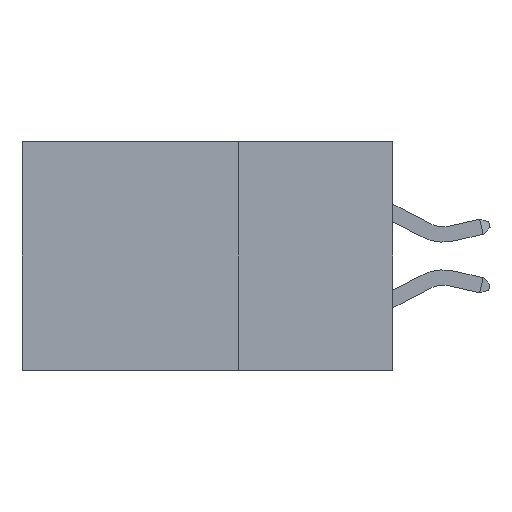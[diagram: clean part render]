
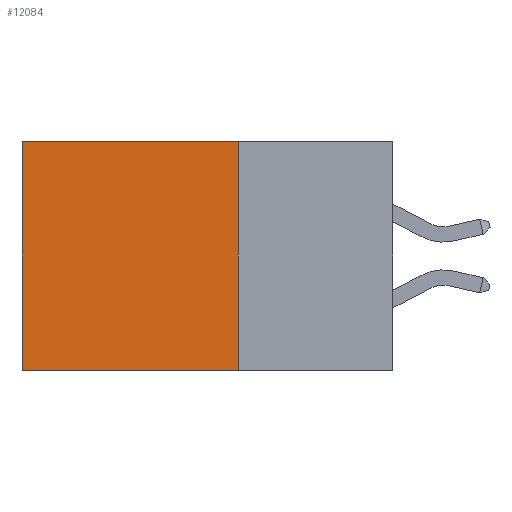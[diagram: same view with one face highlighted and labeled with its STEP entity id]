
A CAD part, left-side view. The second image highlights one B-rep face of the part: STEP entity #12084.
In plain terms, the highlighted planar face has unit normal (-1, 0, 0).
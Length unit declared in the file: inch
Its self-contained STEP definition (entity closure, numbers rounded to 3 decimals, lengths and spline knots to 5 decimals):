
#141 = EDGE_LOOP ( 'NONE', ( #386, #8618, #1111, #3936 ) ) ;
#386 = ORIENTED_EDGE ( 'NONE', *, *, #18227, .T. ) ;
#1111 = ORIENTED_EDGE ( 'NONE', *, *, #12912, .F. ) ;
#1477 = CARTESIAN_POINT ( 'NONE',  ( 0.2875, 0.6, 0. ) ) ;
#1479 = VECTOR ( 'NONE', #14440, 39.37008 ) ;
#1593 = CARTESIAN_POINT ( 'NONE',  ( 0.2875, 0.25, -0.37 ) ) ;
#1992 = LINE ( 'NONE', #6224, #3569 ) ;
#2134 = DIRECTION ( 'NONE',  ( 0., 0., -1. ) ) ;
#2833 = VERTEX_POINT ( 'NONE', #4055 ) ;
#2964 = DIRECTION ( 'NONE',  ( 0., 0., -1. ) ) ;
#3569 = VECTOR ( 'NONE', #8891, 39.37008 ) ;
#3936 = ORIENTED_EDGE ( 'NONE', *, *, #6190, .T. ) ;
#4055 = CARTESIAN_POINT ( 'NONE',  ( 0.2875, 0.25, -0.37 ) ) ;
#4176 = VERTEX_POINT ( 'NONE', #17079 ) ;
#5473 = VECTOR ( 'NONE', #17523, 39.37008 ) ;
#5775 = VECTOR ( 'NONE', #2964, 39.37008 ) ;
#6190 = EDGE_CURVE ( 'NONE', #16853, #18453, #17291, .T. ) ;
#6208 = CARTESIAN_POINT ( 'NONE',  ( 0.2875, 0.25, 0. ) ) ;
#6224 = CARTESIAN_POINT ( 'NONE',  ( 0.2875, 0.25, 0. ) ) ;
#6998 = EDGE_CURVE ( 'NONE', #2833, #4176, #14677, .T. ) ;
#8618 = ORIENTED_EDGE ( 'NONE', *, *, #6998, .F. ) ;
#8865 = DIRECTION ( 'NONE',  ( 1., 0., 0. ) ) ;
#8891 = DIRECTION ( 'NONE',  ( 0., 0., -1. ) ) ;
#9554 = CARTESIAN_POINT ( 'NONE',  ( 0.2875, 0.6, 0. ) ) ;
#10136 = CARTESIAN_POINT ( 'NONE',  ( 0.2875, 0.25, 0. ) ) ;
#12084 = ADVANCED_FACE ( 'NONE', ( #15921 ), #12988, .F. ) ;
#12912 = EDGE_CURVE ( 'NONE', #16853, #2833, #1992, .T. ) ;
#12988 = PLANE ( 'NONE',  #15590 ) ;
#14382 = LINE ( 'NONE', #1477, #5775 ) ;
#14440 = DIRECTION ( 'NONE',  ( 0., 1., 0. ) ) ;
#14677 = LINE ( 'NONE', #1593, #5473 ) ;
#15046 = CARTESIAN_POINT ( 'NONE',  ( 0.2875, 0.25, 0. ) ) ;
#15590 = AXIS2_PLACEMENT_3D ( 'NONE', #15046, #8865, #2134 ) ;
#15921 = FACE_OUTER_BOUND ( 'NONE', #141, .T. ) ;
#16853 = VERTEX_POINT ( 'NONE', #6208 ) ;
#17079 = CARTESIAN_POINT ( 'NONE',  ( 0.2875, 0.6, -0.37 ) ) ;
#17291 = LINE ( 'NONE', #10136, #1479 ) ;
#17523 = DIRECTION ( 'NONE',  ( 0., 1., 0. ) ) ;
#18227 = EDGE_CURVE ( 'NONE', #18453, #4176, #14382, .T. ) ;
#18453 = VERTEX_POINT ( 'NONE', #9554 ) ;
